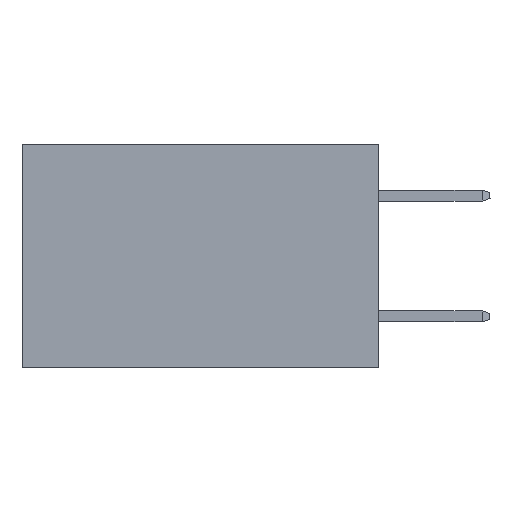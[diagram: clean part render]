
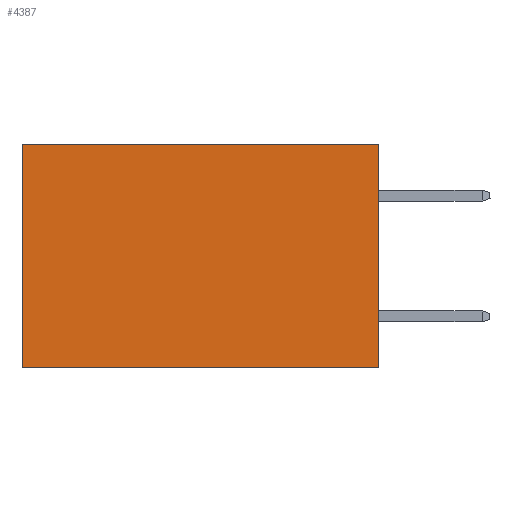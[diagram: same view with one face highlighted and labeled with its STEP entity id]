
A CAD part, left-side view. The second image highlights one B-rep face of the part: STEP entity #4387.
In plain terms, the highlighted planar face has unit normal (-1, 0, 0).
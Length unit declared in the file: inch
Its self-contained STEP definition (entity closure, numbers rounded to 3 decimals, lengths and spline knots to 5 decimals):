
#477 = VERTEX_POINT ( 'NONE', #15010 ) ;
#1048 = CARTESIAN_POINT ( 'NONE',  ( 0.277, 0.59, 0. ) ) ;
#1384 = EDGE_CURVE ( 'NONE', #1587, #7167, #19902, .T. ) ;
#1544 = LINE ( 'NONE', #2575, #27823 ) ;
#1587 = VERTEX_POINT ( 'NONE', #1048 ) ;
#1752 = AXIS2_PLACEMENT_3D ( 'NONE', #26060, #20214, #19553 ) ;
#1807 = CARTESIAN_POINT ( 'NONE',  ( 0.277, 0., -0.37 ) ) ;
#1894 = CARTESIAN_POINT ( 'NONE',  ( 0.277, 0., 0. ) ) ;
#2575 = CARTESIAN_POINT ( 'NONE',  ( 0.277, 0., -0.37 ) ) ;
#3036 = DIRECTION ( 'NONE',  ( 0., 0., -1. ) ) ;
#3965 = CARTESIAN_POINT ( 'NONE',  ( 0.277, 0.59, -0.37 ) ) ;
#4387 = ADVANCED_FACE ( 'NONE', ( #21254 ), #20505, .F. ) ;
#5520 = VECTOR ( 'NONE', #24582, 39.37008 ) ;
#6996 = LINE ( 'NONE', #10745, #26461 ) ;
#7167 = VERTEX_POINT ( 'NONE', #7790 ) ;
#7790 = CARTESIAN_POINT ( 'NONE',  ( 0.277, 0.59, -0.37 ) ) ;
#8709 = ORIENTED_EDGE ( 'NONE', *, *, #25264, .F. ) ;
#8807 = LINE ( 'NONE', #1894, #14005 ) ;
#10745 = CARTESIAN_POINT ( 'NONE',  ( 0.277, 0., -0.37 ) ) ;
#12058 = ORIENTED_EDGE ( 'NONE', *, *, #20897, .T. ) ;
#12871 = DIRECTION ( 'NONE',  ( 0., 1., 0. ) ) ;
#13291 = ORIENTED_EDGE ( 'NONE', *, *, #18512, .F. ) ;
#14005 = VECTOR ( 'NONE', #32292, 39.37008 ) ;
#15010 = CARTESIAN_POINT ( 'NONE',  ( 0.277, 0., 0. ) ) ;
#18512 = EDGE_CURVE ( 'NONE', #477, #25021, #6996, .T. ) ;
#19553 = DIRECTION ( 'NONE',  ( 0., 0., -1. ) ) ;
#19902 = LINE ( 'NONE', #3965, #5520 ) ;
#20214 = DIRECTION ( 'NONE',  ( 1., 0., 0. ) ) ;
#20505 = PLANE ( 'NONE',  #1752 ) ;
#20897 = EDGE_CURVE ( 'NONE', #477, #1587, #8807, .T. ) ;
#21254 = FACE_OUTER_BOUND ( 'NONE', #24687, .T. ) ;
#23248 = ORIENTED_EDGE ( 'NONE', *, *, #1384, .T. ) ;
#24582 = DIRECTION ( 'NONE',  ( 0., 0., -1. ) ) ;
#24687 = EDGE_LOOP ( 'NONE', ( #23248, #8709, #13291, #12058 ) ) ;
#25021 = VERTEX_POINT ( 'NONE', #1807 ) ;
#25264 = EDGE_CURVE ( 'NONE', #25021, #7167, #1544, .T. ) ;
#26060 = CARTESIAN_POINT ( 'NONE',  ( 0.277, 0., -0.37 ) ) ;
#26461 = VECTOR ( 'NONE', #3036, 39.37008 ) ;
#27823 = VECTOR ( 'NONE', #12871, 39.37008 ) ;
#32292 = DIRECTION ( 'NONE',  ( 0., 1., 0. ) ) ;
